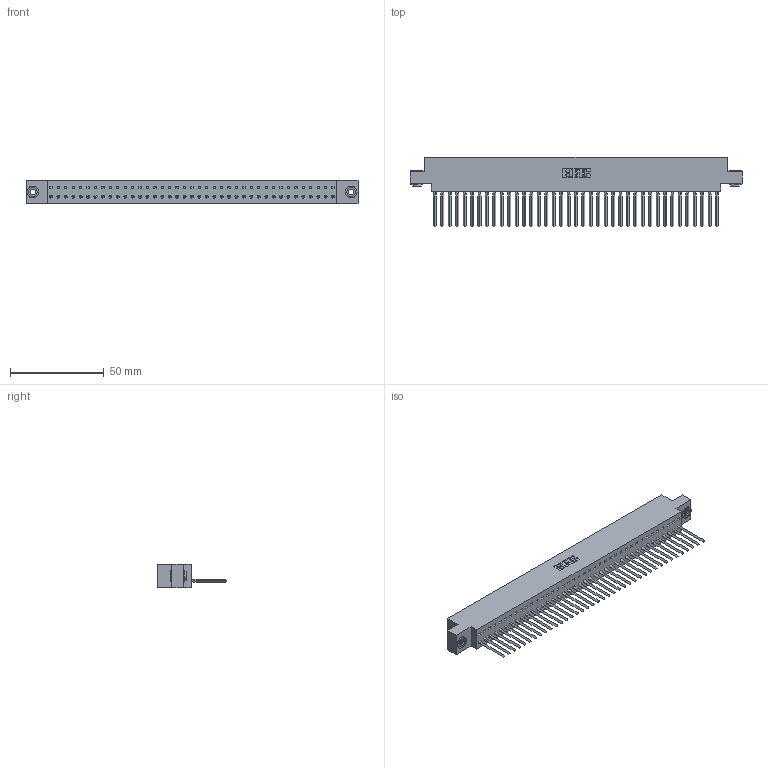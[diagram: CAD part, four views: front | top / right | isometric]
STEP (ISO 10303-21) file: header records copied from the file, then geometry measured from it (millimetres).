
FILE_DESCRIPTION (( 'STEP AP203' ), '1' );
FILE_NAME ('317-039-541-603.STEP', '2020-02-28T00:03:56', ( '' ), ( '' ), 'SwSTEP 2.0', 'SolidWorks 2016', '' );
FILE_SCHEMA (( 'CONFIG_CONTROL_DESIGN' ));
Length unit declared in the file: inch
Products named in the file (4): 317 Part_.156 Dia - TH; 317-290-002_541; 317-039-541-603; 345-250-002_345-250-002-102
Assembly tree (42 placements, depth 2):
  317-039-541-603
    317 Part_.156 Dia - TH
    317-290-002_541  x39
    345-250-002_345-250-002-102  x2
Bounding box: 177.24 x 37.34 x 12.7 mm (x, y, z)
Volume: 28669.7 mm3; surface area: 40626.9 mm2
Topology: 42 solids, 42 shells, 6068 faces, 17277 edges, 11228 vertices
Faces by surface type: plane 4904, cylinder 1000, bspline 156, cone 8
Entity records: 57743 total; most frequent: CARTESIAN_POINT 10873, ORIENTED_EDGE 10158, DIRECTION 8383, EDGE_CURVE 5079, VECTOR 4691, LINE 4691, VERTEX_POINT 3376, AXIS2_PLACEMENT_3D 1846
